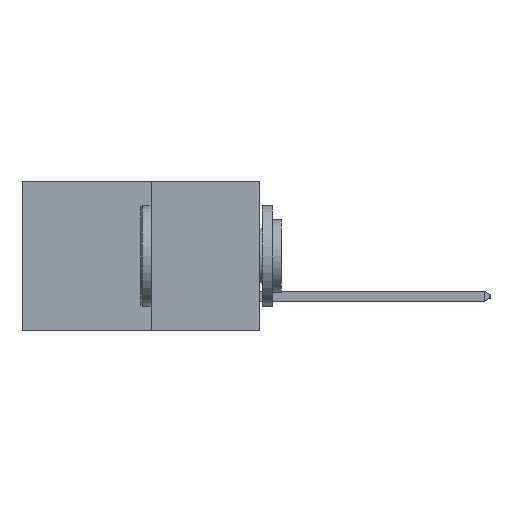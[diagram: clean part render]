
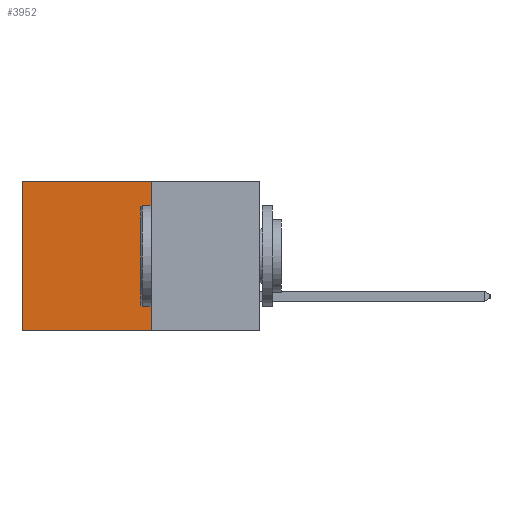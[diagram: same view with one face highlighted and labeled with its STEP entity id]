
A CAD part, left-side view. The second image highlights one B-rep face of the part: STEP entity #3952.
In plain terms, the highlighted planar face has unit normal (-1, 0, 0).
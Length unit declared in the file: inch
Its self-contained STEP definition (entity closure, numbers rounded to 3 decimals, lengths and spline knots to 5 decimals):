
#310 = ORIENTED_EDGE ( 'NONE', *, *, #13216, .F. ) ;
#1537 = CARTESIAN_POINT ( 'NONE',  ( 0.277, 0.59, 0. ) ) ;
#1733 = ORIENTED_EDGE ( 'NONE', *, *, #17122, .F. ) ;
#3952 = ADVANCED_FACE ( 'NONE', ( #4742 ), #11116, .F. ) ;
#4742 = FACE_OUTER_BOUND ( 'NONE', #11825, .T. ) ;
#4778 = CARTESIAN_POINT ( 'NONE',  ( 0.277, 0.59, -0.37 ) ) ;
#5679 = VERTEX_POINT ( 'NONE', #1537 ) ;
#5994 = VERTEX_POINT ( 'NONE', #18433 ) ;
#7208 = EDGE_CURVE ( 'NONE', #5994, #5679, #8503, .T. ) ;
#8354 = LINE ( 'NONE', #25859, #24479 ) ;
#8503 = LINE ( 'NONE', #14303, #23997 ) ;
#9695 = CARTESIAN_POINT ( 'NONE',  ( 0.277, 0.59, -0.37 ) ) ;
#10084 = DIRECTION ( 'NONE',  ( 0., 0., -1. ) ) ;
#10170 = DIRECTION ( 'NONE',  ( 1., 0., 0. ) ) ;
#10694 = EDGE_CURVE ( 'NONE', #5679, #12474, #15453, .T. ) ;
#11116 = PLANE ( 'NONE',  #16499 ) ;
#11210 = DIRECTION ( 'NONE',  ( 0., 1., 0. ) ) ;
#11478 = DIRECTION ( 'NONE',  ( 0., 0., -1. ) ) ;
#11760 = CARTESIAN_POINT ( 'NONE',  ( 0.277, 0.27, -0.37 ) ) ;
#11825 = EDGE_LOOP ( 'NONE', ( #17091, #1733, #310, #15587 ) ) ;
#12313 = LINE ( 'NONE', #24092, #23506 ) ;
#12474 = VERTEX_POINT ( 'NONE', #4778 ) ;
#13216 = EDGE_CURVE ( 'NONE', #5994, #16407, #12313, .T. ) ;
#14182 = DIRECTION ( 'NONE',  ( 0., 1., 0. ) ) ;
#14303 = CARTESIAN_POINT ( 'NONE',  ( 0.277, 0.27, 0. ) ) ;
#15436 = CARTESIAN_POINT ( 'NONE',  ( 0.277, 0.27, -0.37 ) ) ;
#15453 = LINE ( 'NONE', #9695, #21060 ) ;
#15587 = ORIENTED_EDGE ( 'NONE', *, *, #7208, .T. ) ;
#16407 = VERTEX_POINT ( 'NONE', #15436 ) ;
#16499 = AXIS2_PLACEMENT_3D ( 'NONE', #11760, #10170, #10084 ) ;
#17091 = ORIENTED_EDGE ( 'NONE', *, *, #10694, .T. ) ;
#17122 = EDGE_CURVE ( 'NONE', #16407, #12474, #8354, .T. ) ;
#18433 = CARTESIAN_POINT ( 'NONE',  ( 0.277, 0.27, 0. ) ) ;
#21060 = VECTOR ( 'NONE', #24410, 39.37008 ) ;
#23506 = VECTOR ( 'NONE', #11478, 39.37008 ) ;
#23997 = VECTOR ( 'NONE', #14182, 39.37008 ) ;
#24092 = CARTESIAN_POINT ( 'NONE',  ( 0.277, 0.27, -0.37 ) ) ;
#24410 = DIRECTION ( 'NONE',  ( 0., 0., -1. ) ) ;
#24479 = VECTOR ( 'NONE', #11210, 39.37008 ) ;
#25859 = CARTESIAN_POINT ( 'NONE',  ( 0.277, 0.27, -0.37 ) ) ;
